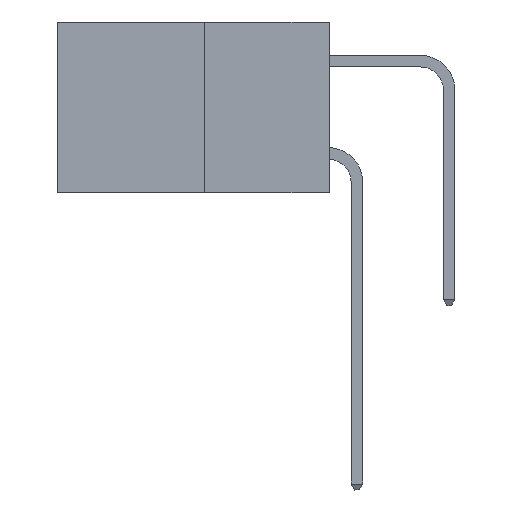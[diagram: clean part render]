
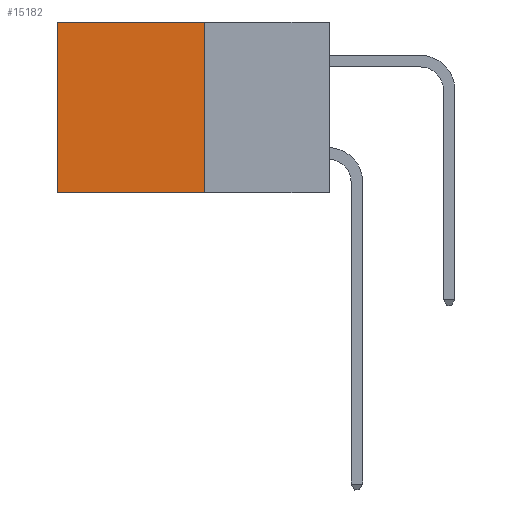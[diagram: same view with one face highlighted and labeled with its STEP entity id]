
A CAD part, left-side view. The second image highlights one B-rep face of the part: STEP entity #15182.
In plain terms, the highlighted planar face has unit normal (-1, 0, 0).
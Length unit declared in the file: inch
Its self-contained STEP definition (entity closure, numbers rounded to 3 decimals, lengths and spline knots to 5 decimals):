
#72 = PLANE ( 'NONE',  #23460 ) ;
#638 = VERTEX_POINT ( 'NONE', #12966 ) ;
#669 = VERTEX_POINT ( 'NONE', #5298 ) ;
#1912 = DIRECTION ( 'NONE',  ( 0., 0., -1. ) ) ;
#2438 = LINE ( 'NONE', #16626, #5631 ) ;
#2634 = VERTEX_POINT ( 'NONE', #16066 ) ;
#4044 = CARTESIAN_POINT ( 'NONE',  ( 0.277, 0.27, -0.37 ) ) ;
#4131 = DIRECTION ( 'NONE',  ( 0., 0., -1. ) ) ;
#5081 = CARTESIAN_POINT ( 'NONE',  ( 0.277, 0.27, 0. ) ) ;
#5240 = DIRECTION ( 'NONE',  ( 0., 1., 0. ) ) ;
#5298 = CARTESIAN_POINT ( 'NONE',  ( 0.277, 0.27, 0. ) ) ;
#5631 = VECTOR ( 'NONE', #20349, 39.37008 ) ;
#7346 = VECTOR ( 'NONE', #12471, 39.37008 ) ;
#9483 = ORIENTED_EDGE ( 'NONE', *, *, #17518, .F. ) ;
#9635 = ORIENTED_EDGE ( 'NONE', *, *, #18976, .F. ) ;
#11357 = CARTESIAN_POINT ( 'NONE',  ( 0.277, 0.59, -0.37 ) ) ;
#11465 = LINE ( 'NONE', #16260, #15187 ) ;
#12471 = DIRECTION ( 'NONE',  ( 0., 1., 0. ) ) ;
#12736 = FACE_OUTER_BOUND ( 'NONE', #17559, .T. ) ;
#12935 = DIRECTION ( 'NONE',  ( 1., 0., 0. ) ) ;
#12966 = CARTESIAN_POINT ( 'NONE',  ( 0.277, 0.59, 0. ) ) ;
#13240 = LINE ( 'NONE', #4044, #22362 ) ;
#13921 = EDGE_CURVE ( 'NONE', #638, #21067, #2438, .T. ) ;
#14864 = ORIENTED_EDGE ( 'NONE', *, *, #20868, .T. ) ;
#15182 = ADVANCED_FACE ( 'NONE', ( #12736 ), #72, .F. ) ;
#15187 = VECTOR ( 'NONE', #5240, 39.37008 ) ;
#16066 = CARTESIAN_POINT ( 'NONE',  ( 0.277, 0.27, -0.37 ) ) ;
#16260 = CARTESIAN_POINT ( 'NONE',  ( 0.277, 0.27, -0.37 ) ) ;
#16626 = CARTESIAN_POINT ( 'NONE',  ( 0.277, 0.59, -0.37 ) ) ;
#17518 = EDGE_CURVE ( 'NONE', #669, #2634, #13240, .T. ) ;
#17559 = EDGE_LOOP ( 'NONE', ( #18492, #9635, #9483, #14864 ) ) ;
#17694 = LINE ( 'NONE', #5081, #7346 ) ;
#18492 = ORIENTED_EDGE ( 'NONE', *, *, #13921, .T. ) ;
#18976 = EDGE_CURVE ( 'NONE', #2634, #21067, #11465, .T. ) ;
#20227 = CARTESIAN_POINT ( 'NONE',  ( 0.277, 0.27, -0.37 ) ) ;
#20349 = DIRECTION ( 'NONE',  ( 0., 0., -1. ) ) ;
#20868 = EDGE_CURVE ( 'NONE', #669, #638, #17694, .T. ) ;
#21067 = VERTEX_POINT ( 'NONE', #11357 ) ;
#22362 = VECTOR ( 'NONE', #4131, 39.37008 ) ;
#23460 = AXIS2_PLACEMENT_3D ( 'NONE', #20227, #12935, #1912 ) ;
